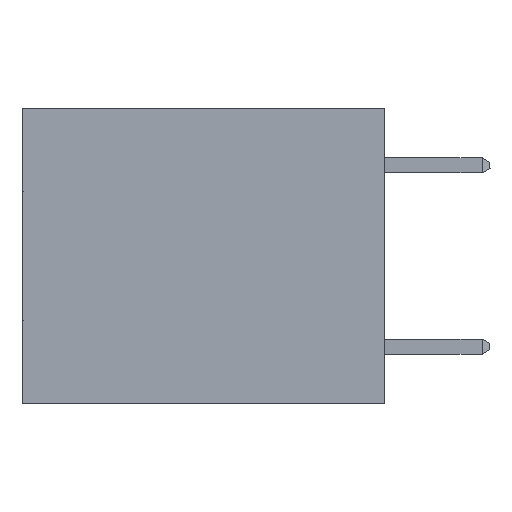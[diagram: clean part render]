
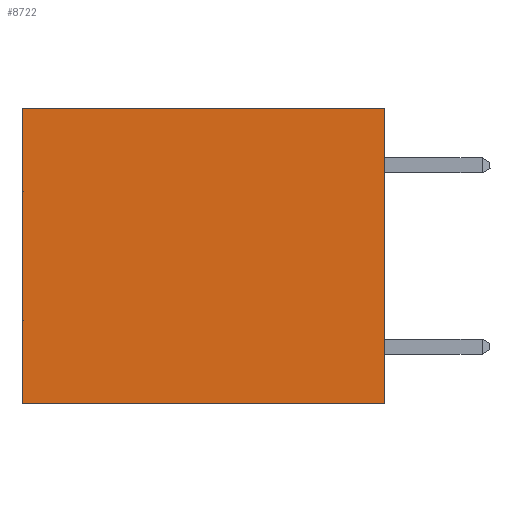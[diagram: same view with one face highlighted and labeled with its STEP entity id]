
A CAD part, left-side view. The second image highlights one B-rep face of the part: STEP entity #8722.
In plain terms, the highlighted planar face has unit normal (-1, 0, 0).
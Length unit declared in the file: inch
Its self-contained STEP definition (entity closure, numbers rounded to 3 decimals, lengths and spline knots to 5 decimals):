
#681 = CARTESIAN_POINT ( 'NONE',  ( 0.3165, 0.6, 0. ) ) ;
#4565 = CARTESIAN_POINT ( 'NONE',  ( 0.3165, 0., -0.49 ) ) ;
#5229 = CARTESIAN_POINT ( 'NONE',  ( 0.3165, 0.6, -0.49 ) ) ;
#5602 = DIRECTION ( 'NONE',  ( 0., 0., -1. ) ) ;
#5986 = LINE ( 'NONE', #21788, #12912 ) ;
#6423 = AXIS2_PLACEMENT_3D ( 'NONE', #26475, #13947, #10990 ) ;
#8240 = PLANE ( 'NONE',  #6423 ) ;
#8722 = ADVANCED_FACE ( 'NONE', ( #30777 ), #8240, .F. ) ;
#9343 = ORIENTED_EDGE ( 'NONE', *, *, #21216, .F. ) ;
#10061 = VERTEX_POINT ( 'NONE', #681 ) ;
#10863 = DIRECTION ( 'NONE',  ( 0., 1., 0. ) ) ;
#10990 = DIRECTION ( 'NONE',  ( 0., 0., -1. ) ) ;
#11936 = EDGE_CURVE ( 'NONE', #27061, #17689, #5986, .T. ) ;
#12625 = VECTOR ( 'NONE', #22641, 39.37008 ) ;
#12912 = VECTOR ( 'NONE', #5602, 39.37008 ) ;
#13648 = CARTESIAN_POINT ( 'NONE',  ( 0.3165, 0., 0. ) ) ;
#13947 = DIRECTION ( 'NONE',  ( 1., 0., 0. ) ) ;
#16561 = DIRECTION ( 'NONE',  ( 0., 0., -1. ) ) ;
#17689 = VERTEX_POINT ( 'NONE', #4565 ) ;
#18965 = ORIENTED_EDGE ( 'NONE', *, *, #11936, .F. ) ;
#19984 = LINE ( 'NONE', #33867, #12625 ) ;
#20019 = VECTOR ( 'NONE', #10863, 39.37008 ) ;
#20258 = LINE ( 'NONE', #24226, #31361 ) ;
#21150 = CARTESIAN_POINT ( 'NONE',  ( 0.3165, 0., -0.49 ) ) ;
#21216 = EDGE_CURVE ( 'NONE', #17689, #24023, #27853, .T. ) ;
#21788 = CARTESIAN_POINT ( 'NONE',  ( 0.3165, 0., -0.49 ) ) ;
#22641 = DIRECTION ( 'NONE',  ( 0., 1., 0. ) ) ;
#23383 = EDGE_CURVE ( 'NONE', #10061, #24023, #20258, .T. ) ;
#24023 = VERTEX_POINT ( 'NONE', #5229 ) ;
#24226 = CARTESIAN_POINT ( 'NONE',  ( 0.3165, 0.6, -0.49 ) ) ;
#26475 = CARTESIAN_POINT ( 'NONE',  ( 0.3165, 0., -0.49 ) ) ;
#27061 = VERTEX_POINT ( 'NONE', #13648 ) ;
#27853 = LINE ( 'NONE', #21150, #20019 ) ;
#28810 = ORIENTED_EDGE ( 'NONE', *, *, #32915, .T. ) ;
#29733 = EDGE_LOOP ( 'NONE', ( #31093, #9343, #18965, #28810 ) ) ;
#30777 = FACE_OUTER_BOUND ( 'NONE', #29733, .T. ) ;
#31093 = ORIENTED_EDGE ( 'NONE', *, *, #23383, .T. ) ;
#31361 = VECTOR ( 'NONE', #16561, 39.37008 ) ;
#32915 = EDGE_CURVE ( 'NONE', #27061, #10061, #19984, .T. ) ;
#33867 = CARTESIAN_POINT ( 'NONE',  ( 0.3165, 0., 0. ) ) ;
